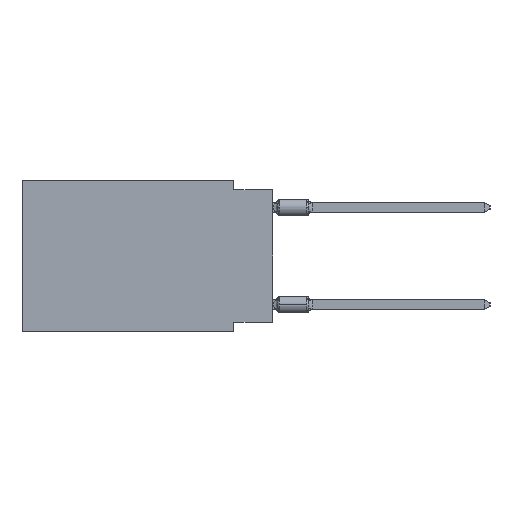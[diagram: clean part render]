
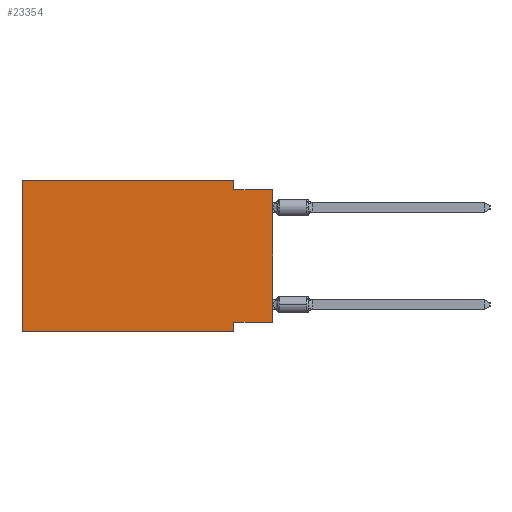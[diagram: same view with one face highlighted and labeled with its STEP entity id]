
A CAD part, left-side view. The second image highlights one B-rep face of the part: STEP entity #23354.
In plain terms, the highlighted planar face has unit normal (-1, 0, 0).
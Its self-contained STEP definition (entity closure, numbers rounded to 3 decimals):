
#304 = VERTEX_POINT ( 'NONE', #22300 ) ;
#356 = EDGE_CURVE ( 'NONE', #26631, #21192, #15678, .T. ) ;
#959 = CARTESIAN_POINT ( 'NONE',  ( 0., 0., -0.635 ) ) ;
#989 = DIRECTION ( 'NONE',  ( 0., 0., 1. ) ) ;
#1002 = CARTESIAN_POINT ( 'NONE',  ( 0., 2.54, -0.635 ) ) ;
#1132 = DIRECTION ( 'NONE',  ( 1., 0., 0. ) ) ;
#1451 = CARTESIAN_POINT ( 'NONE',  ( 0., 2.54, -9.906 ) ) ;
#1924 = LINE ( 'NONE', #1451, #6552 ) ;
#3206 = CARTESIAN_POINT ( 'NONE',  ( 0., 16.383, 0. ) ) ;
#3943 = CARTESIAN_POINT ( 'NONE',  ( 0., 2.54, 0. ) ) ;
#4701 = ORIENTED_EDGE ( 'NONE', *, *, #30410, .T. ) ;
#5576 = CARTESIAN_POINT ( 'NONE',  ( 0., 16.383, 0. ) ) ;
#5585 = LINE ( 'NONE', #3206, #7397 ) ;
#5813 = LINE ( 'NONE', #22365, #19500 ) ;
#5854 = LINE ( 'NONE', #959, #15197 ) ;
#6552 = VECTOR ( 'NONE', #11075, 1000. ) ;
#6569 = LINE ( 'NONE', #28642, #16078 ) ;
#6734 = CARTESIAN_POINT ( 'NONE',  ( 0., 0., -9.271 ) ) ;
#7397 = VECTOR ( 'NONE', #29404, 1000. ) ;
#8371 = DIRECTION ( 'NONE',  ( 0., -1., 0. ) ) ;
#8481 = CARTESIAN_POINT ( 'NONE',  ( 0., 16.383, -9.906 ) ) ;
#9103 = LINE ( 'NONE', #20936, #14883 ) ;
#9275 = ORIENTED_EDGE ( 'NONE', *, *, #27478, .F. ) ;
#9389 = VERTEX_POINT ( 'NONE', #25937 ) ;
#10595 = DIRECTION ( 'NONE',  ( 0., 0., -1. ) ) ;
#10657 = EDGE_CURVE ( 'NONE', #23883, #15299, #9103, .T. ) ;
#11075 = DIRECTION ( 'NONE',  ( 0., 0., -1. ) ) ;
#11478 = AXIS2_PLACEMENT_3D ( 'NONE', #5576, #1132, #10595 ) ;
#12511 = EDGE_CURVE ( 'NONE', #26631, #9389, #5585, .T. ) ;
#12941 = EDGE_CURVE ( 'NONE', #9389, #23883, #5813, .T. ) ;
#12955 = LINE ( 'NONE', #22590, #21866 ) ;
#14883 = VECTOR ( 'NONE', #23140, 1000. ) ;
#15059 = EDGE_CURVE ( 'NONE', #19890, #304, #6569, .T. ) ;
#15197 = VECTOR ( 'NONE', #8371, 1000. ) ;
#15299 = VERTEX_POINT ( 'NONE', #1002 ) ;
#15678 = LINE ( 'NONE', #25295, #29808 ) ;
#16078 = VECTOR ( 'NONE', #16640, 1000. ) ;
#16366 = ORIENTED_EDGE ( 'NONE', *, *, #15059, .F. ) ;
#16640 = DIRECTION ( 'NONE',  ( 0., 1., 0. ) ) ;
#17044 = ORIENTED_EDGE ( 'NONE', *, *, #24593, .F. ) ;
#17574 = DIRECTION ( 'NONE',  ( 0., -1., 0. ) ) ;
#18021 = EDGE_LOOP ( 'NONE', ( #4701, #9275, #26804, #21092, #28376, #26496, #17044, #16366 ) ) ;
#19500 = VECTOR ( 'NONE', #30104, 1000. ) ;
#19890 = VERTEX_POINT ( 'NONE', #6734 ) ;
#20936 = CARTESIAN_POINT ( 'NONE',  ( 0., 2.54, 0. ) ) ;
#21092 = ORIENTED_EDGE ( 'NONE', *, *, #12941, .F. ) ;
#21192 = VERTEX_POINT ( 'NONE', #31047 ) ;
#21866 = VECTOR ( 'NONE', #989, 1000. ) ;
#22300 = CARTESIAN_POINT ( 'NONE',  ( 0., 2.54, -9.271 ) ) ;
#22365 = CARTESIAN_POINT ( 'NONE',  ( 0., 16.383, 0. ) ) ;
#22590 = CARTESIAN_POINT ( 'NONE',  ( 0., 0., 0. ) ) ;
#23140 = DIRECTION ( 'NONE',  ( 0., 0., -1. ) ) ;
#23354 = ADVANCED_FACE ( 'NONE', ( #29391 ), #24648, .F. ) ;
#23883 = VERTEX_POINT ( 'NONE', #3943 ) ;
#24593 = EDGE_CURVE ( 'NONE', #304, #21192, #1924, .T. ) ;
#24648 = PLANE ( 'NONE',  #11478 ) ;
#25295 = CARTESIAN_POINT ( 'NONE',  ( 0., 16.383, -9.906 ) ) ;
#25937 = CARTESIAN_POINT ( 'NONE',  ( 0., 16.383, 0. ) ) ;
#26496 = ORIENTED_EDGE ( 'NONE', *, *, #356, .T. ) ;
#26631 = VERTEX_POINT ( 'NONE', #8481 ) ;
#26804 = ORIENTED_EDGE ( 'NONE', *, *, #10657, .F. ) ;
#27478 = EDGE_CURVE ( 'NONE', #15299, #29494, #5854, .T. ) ;
#28267 = CARTESIAN_POINT ( 'NONE',  ( 0., 0., -0.635 ) ) ;
#28376 = ORIENTED_EDGE ( 'NONE', *, *, #12511, .F. ) ;
#28642 = CARTESIAN_POINT ( 'NONE',  ( 0., 0., -9.271 ) ) ;
#29391 = FACE_OUTER_BOUND ( 'NONE', #18021, .T. ) ;
#29404 = DIRECTION ( 'NONE',  ( 0., 0., 1. ) ) ;
#29494 = VERTEX_POINT ( 'NONE', #28267 ) ;
#29808 = VECTOR ( 'NONE', #17574, 1000. ) ;
#30104 = DIRECTION ( 'NONE',  ( 0., -1., 0. ) ) ;
#30410 = EDGE_CURVE ( 'NONE', #19890, #29494, #12955, .T. ) ;
#31047 = CARTESIAN_POINT ( 'NONE',  ( 0., 2.54, -9.906 ) ) ;
